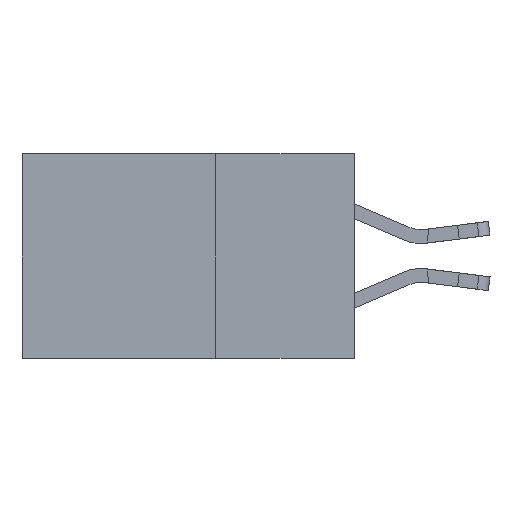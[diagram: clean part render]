
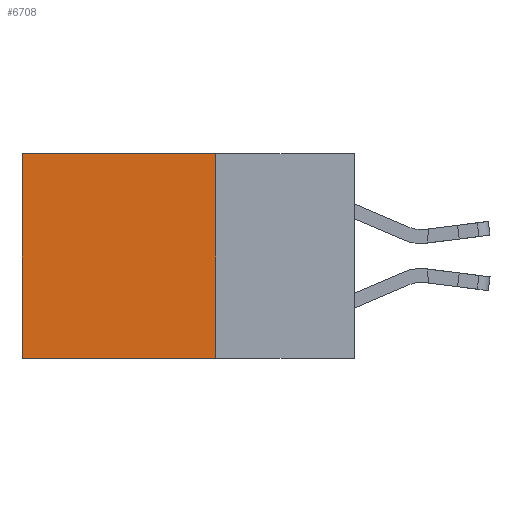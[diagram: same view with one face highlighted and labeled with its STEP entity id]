
A CAD part, left-side view. The second image highlights one B-rep face of the part: STEP entity #6708.
In plain terms, the highlighted planar face has unit normal (-1, 0, 0).
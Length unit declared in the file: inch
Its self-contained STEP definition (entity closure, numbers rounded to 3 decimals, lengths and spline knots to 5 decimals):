
#963 = ORIENTED_EDGE ( 'NONE', *, *, #18601, .F. ) ;
#2087 = CARTESIAN_POINT ( 'NONE',  ( 0.2615, 0.25, 0. ) ) ;
#3133 = CARTESIAN_POINT ( 'NONE',  ( 0.2615, 0.25, -0.37 ) ) ;
#3222 = EDGE_CURVE ( 'NONE', #19954, #12492, #11538, .T. ) ;
#4271 = VECTOR ( 'NONE', #4777, 39.37008 ) ;
#4777 = DIRECTION ( 'NONE',  ( 0., 1., 0. ) ) ;
#5115 = VERTEX_POINT ( 'NONE', #12154 ) ;
#5596 = CARTESIAN_POINT ( 'NONE',  ( 0.2615, 0.6, -0.37 ) ) ;
#6289 = CARTESIAN_POINT ( 'NONE',  ( 0.2615, 0.25, -0.37 ) ) ;
#6708 = ADVANCED_FACE ( 'NONE', ( #10575 ), #12652, .F. ) ;
#8175 = ORIENTED_EDGE ( 'NONE', *, *, #3222, .F. ) ;
#8432 = CARTESIAN_POINT ( 'NONE',  ( 0.2615, 0.25, -0.37 ) ) ;
#8528 = VERTEX_POINT ( 'NONE', #17539 ) ;
#8843 = DIRECTION ( 'NONE',  ( 0., 0., -1. ) ) ;
#9555 = DIRECTION ( 'NONE',  ( 0., 0., -1. ) ) ;
#9755 = CARTESIAN_POINT ( 'NONE',  ( 0.2615, 0.25, 0. ) ) ;
#10048 = AXIS2_PLACEMENT_3D ( 'NONE', #6289, #18965, #9555 ) ;
#10575 = FACE_OUTER_BOUND ( 'NONE', #12030, .T. ) ;
#11538 = LINE ( 'NONE', #8432, #15251 ) ;
#12030 = EDGE_LOOP ( 'NONE', ( #20169, #963, #8175, #14138 ) ) ;
#12064 = CARTESIAN_POINT ( 'NONE',  ( 0.2615, 0.25, -0.37 ) ) ;
#12154 = CARTESIAN_POINT ( 'NONE',  ( 0.2615, 0.6, -0.37 ) ) ;
#12492 = VERTEX_POINT ( 'NONE', #12064 ) ;
#12652 = PLANE ( 'NONE',  #10048 ) ;
#13283 = LINE ( 'NONE', #3133, #4271 ) ;
#14138 = ORIENTED_EDGE ( 'NONE', *, *, #19784, .T. ) ;
#15251 = VECTOR ( 'NONE', #17079, 39.37008 ) ;
#15472 = EDGE_CURVE ( 'NONE', #8528, #5115, #20453, .T. ) ;
#16653 = LINE ( 'NONE', #9755, #20350 ) ;
#17079 = DIRECTION ( 'NONE',  ( 0., 0., -1. ) ) ;
#17539 = CARTESIAN_POINT ( 'NONE',  ( 0.2615, 0.6, 0. ) ) ;
#18601 = EDGE_CURVE ( 'NONE', #12492, #5115, #13283, .T. ) ;
#18965 = DIRECTION ( 'NONE',  ( 1., 0., 0. ) ) ;
#19147 = DIRECTION ( 'NONE',  ( 0., 1., 0. ) ) ;
#19784 = EDGE_CURVE ( 'NONE', #19954, #8528, #16653, .T. ) ;
#19954 = VERTEX_POINT ( 'NONE', #2087 ) ;
#19963 = VECTOR ( 'NONE', #8843, 39.37008 ) ;
#20169 = ORIENTED_EDGE ( 'NONE', *, *, #15472, .T. ) ;
#20350 = VECTOR ( 'NONE', #19147, 39.37008 ) ;
#20453 = LINE ( 'NONE', #5596, #19963 ) ;
